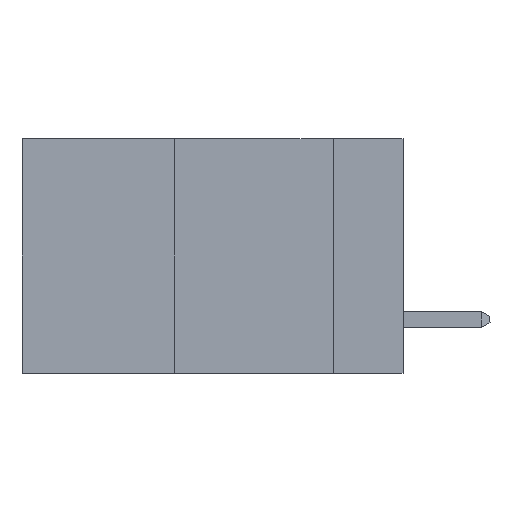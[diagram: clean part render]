
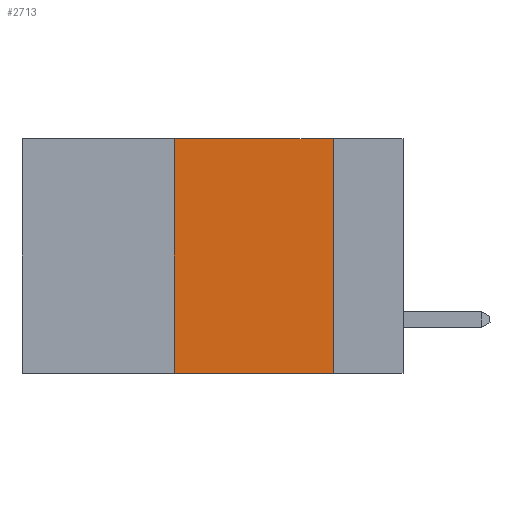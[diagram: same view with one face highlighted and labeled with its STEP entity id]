
A CAD part, left-side view. The second image highlights one B-rep face of the part: STEP entity #2713.
In plain terms, the highlighted planar face has unit normal (-1, 0, 0).
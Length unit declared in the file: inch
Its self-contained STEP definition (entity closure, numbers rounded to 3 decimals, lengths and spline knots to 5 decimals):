
#130 = FACE_OUTER_BOUND ( 'NONE', #2203, .T. ) ;
#134 = CARTESIAN_POINT ( 'NONE',  ( 0., 0.36, 0. ) ) ;
#150 = EDGE_CURVE ( 'NONE', #6261, #3098, #3710, .T. ) ;
#161 = DIRECTION ( 'NONE',  ( 0., 0., -1. ) ) ;
#189 = PLANE ( 'NONE',  #10646 ) ;
#199 = CARTESIAN_POINT ( 'NONE',  ( 0., 0.6, 0. ) ) ;
#303 = DIRECTION ( 'NONE',  ( 1., 0., 0. ) ) ;
#383 = EDGE_CURVE ( 'NONE', #6261, #2884, #2500, .T. ) ;
#576 = ORIENTED_EDGE ( 'NONE', *, *, #9591, .F. ) ;
#609 = ORIENTED_EDGE ( 'NONE', *, *, #8895, .F. ) ;
#824 = DIRECTION ( 'NONE',  ( 0., 0., 1. ) ) ;
#895 = ORIENTED_EDGE ( 'NONE', *, *, #383, .F. ) ;
#924 = CARTESIAN_POINT ( 'NONE',  ( 0., 0.11, -0.37 ) ) ;
#1160 = ORIENTED_EDGE ( 'NONE', *, *, #150, .T. ) ;
#2203 = EDGE_LOOP ( 'NONE', ( #576, #609, #895, #1160 ) ) ;
#2304 = CARTESIAN_POINT ( 'NONE',  ( 0., 0.11, 0. ) ) ;
#2327 = VECTOR ( 'NONE', #4964, 39.37008 ) ;
#2500 = LINE ( 'NONE', #5976, #10463 ) ;
#2713 = ADVANCED_FACE ( 'NONE', ( #130 ), #189, .F. ) ;
#2884 = VERTEX_POINT ( 'NONE', #134 ) ;
#3098 = VERTEX_POINT ( 'NONE', #924 ) ;
#3270 = VERTEX_POINT ( 'NONE', #2304 ) ;
#3710 = LINE ( 'NONE', #6651, #5643 ) ;
#3944 = CARTESIAN_POINT ( 'NONE',  ( 0., 0.36, -0.37 ) ) ;
#4964 = DIRECTION ( 'NONE',  ( 0., 0., -1. ) ) ;
#5643 = VECTOR ( 'NONE', #10733, 39.37008 ) ;
#5976 = CARTESIAN_POINT ( 'NONE',  ( 0., 0.36, 0. ) ) ;
#6261 = VERTEX_POINT ( 'NONE', #3944 ) ;
#6573 = CARTESIAN_POINT ( 'NONE',  ( 0., 0.11, 0. ) ) ;
#6634 = VECTOR ( 'NONE', #7414, 39.37008 ) ;
#6651 = CARTESIAN_POINT ( 'NONE',  ( 0., 0.6, -0.37 ) ) ;
#7414 = DIRECTION ( 'NONE',  ( 0., -1., 0. ) ) ;
#8593 = LINE ( 'NONE', #10356, #6634 ) ;
#8823 = LINE ( 'NONE', #6573, #2327 ) ;
#8895 = EDGE_CURVE ( 'NONE', #2884, #3270, #8593, .T. ) ;
#9591 = EDGE_CURVE ( 'NONE', #3270, #3098, #8823, .T. ) ;
#10356 = CARTESIAN_POINT ( 'NONE',  ( 0., 0.6, 0. ) ) ;
#10463 = VECTOR ( 'NONE', #824, 39.37008 ) ;
#10646 = AXIS2_PLACEMENT_3D ( 'NONE', #199, #303, #161 ) ;
#10733 = DIRECTION ( 'NONE',  ( 0., -1., 0. ) ) ;
